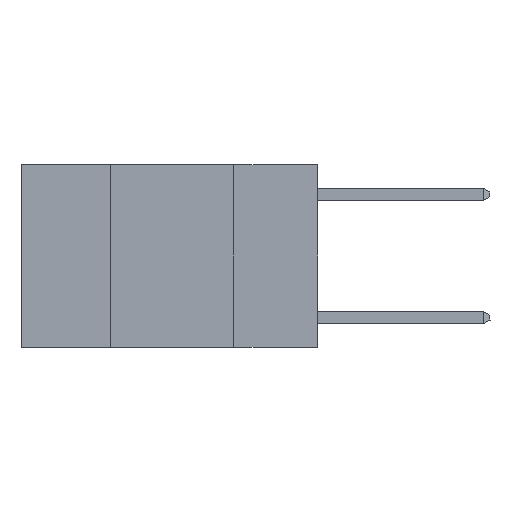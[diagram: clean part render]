
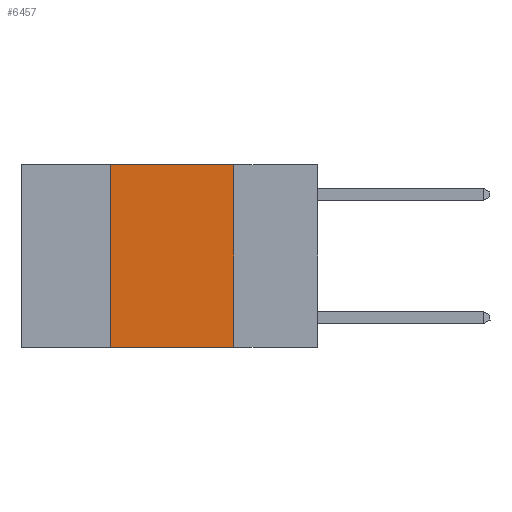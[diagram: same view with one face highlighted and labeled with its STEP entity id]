
A CAD part, left-side view. The second image highlights one B-rep face of the part: STEP entity #6457.
In plain terms, the highlighted planar face has unit normal (-1, 0, 0).
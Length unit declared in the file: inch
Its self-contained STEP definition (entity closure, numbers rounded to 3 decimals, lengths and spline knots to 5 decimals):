
#165 = DIRECTION ( 'NONE',  ( 0., 0., 1. ) ) ;
#804 = LINE ( 'NONE', #5424, #12595 ) ;
#1542 = VERTEX_POINT ( 'NONE', #13708 ) ;
#2100 = CARTESIAN_POINT ( 'NONE',  ( 0., 0.6, 0. ) ) ;
#2347 = CARTESIAN_POINT ( 'NONE',  ( 0., 0.17, -0.37 ) ) ;
#3892 = DIRECTION ( 'NONE',  ( 1., 0., 0. ) ) ;
#5424 = CARTESIAN_POINT ( 'NONE',  ( 0., 0.42, 0. ) ) ;
#6457 = ADVANCED_FACE ( 'NONE', ( #18681 ), #12602, .F. ) ;
#6627 = ORIENTED_EDGE ( 'NONE', *, *, #9952, .F. ) ;
#7424 = DIRECTION ( 'NONE',  ( 0., -1., 0. ) ) ;
#8075 = EDGE_CURVE ( 'NONE', #1542, #9524, #18358, .T. ) ;
#9524 = VERTEX_POINT ( 'NONE', #2347 ) ;
#9567 = DIRECTION ( 'NONE',  ( 0., -1., 0. ) ) ;
#9952 = EDGE_CURVE ( 'NONE', #1542, #14374, #804, .T. ) ;
#10315 = ORIENTED_EDGE ( 'NONE', *, *, #11619, .F. ) ;
#10804 = EDGE_CURVE ( 'NONE', #14374, #14403, #18234, .T. ) ;
#11310 = CARTESIAN_POINT ( 'NONE',  ( 0., 0.17, 0. ) ) ;
#11619 = EDGE_CURVE ( 'NONE', #14403, #9524, #16653, .T. ) ;
#11957 = CARTESIAN_POINT ( 'NONE',  ( 0., 0.42, 0. ) ) ;
#12595 = VECTOR ( 'NONE', #165, 39.37008 ) ;
#12602 = PLANE ( 'NONE',  #21025 ) ;
#12687 = VECTOR ( 'NONE', #7424, 39.37008 ) ;
#12823 = ORIENTED_EDGE ( 'NONE', *, *, #10804, .F. ) ;
#12912 = ORIENTED_EDGE ( 'NONE', *, *, #8075, .T. ) ;
#13055 = DIRECTION ( 'NONE',  ( 0., 0., -1. ) ) ;
#13708 = CARTESIAN_POINT ( 'NONE',  ( 0., 0.42, -0.37 ) ) ;
#14374 = VERTEX_POINT ( 'NONE', #11957 ) ;
#14403 = VERTEX_POINT ( 'NONE', #17268 ) ;
#16121 = DIRECTION ( 'NONE',  ( 0., 0., -1. ) ) ;
#16653 = LINE ( 'NONE', #11310, #20561 ) ;
#17268 = CARTESIAN_POINT ( 'NONE',  ( 0., 0.17, 0. ) ) ;
#18234 = LINE ( 'NONE', #19841, #22117 ) ;
#18358 = LINE ( 'NONE', #19512, #12687 ) ;
#18681 = FACE_OUTER_BOUND ( 'NONE', #21063, .T. ) ;
#19512 = CARTESIAN_POINT ( 'NONE',  ( 0., 0.6, -0.37 ) ) ;
#19841 = CARTESIAN_POINT ( 'NONE',  ( 0., 0.6, 0. ) ) ;
#20561 = VECTOR ( 'NONE', #13055, 39.37008 ) ;
#21025 = AXIS2_PLACEMENT_3D ( 'NONE', #2100, #3892, #16121 ) ;
#21063 = EDGE_LOOP ( 'NONE', ( #10315, #12823, #6627, #12912 ) ) ;
#22117 = VECTOR ( 'NONE', #9567, 39.37008 ) ;
